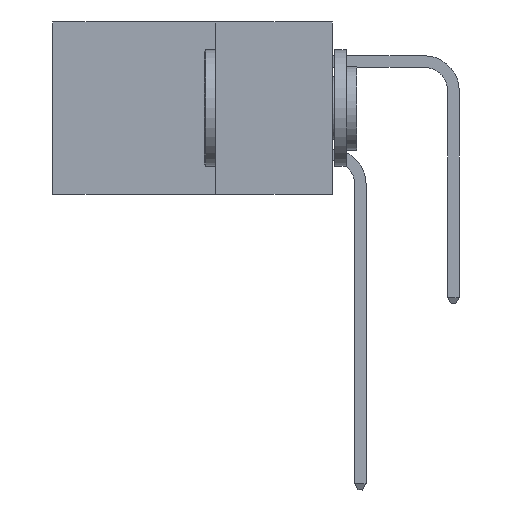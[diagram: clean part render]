
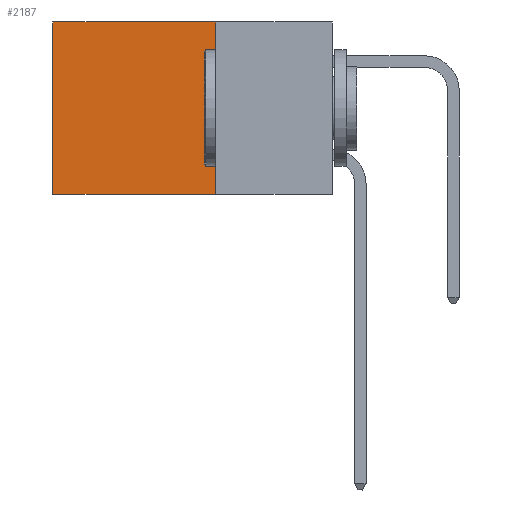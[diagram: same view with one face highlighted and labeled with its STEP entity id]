
A CAD part, left-side view. The second image highlights one B-rep face of the part: STEP entity #2187.
In plain terms, the highlighted planar face has unit normal (-1, 0, 0).
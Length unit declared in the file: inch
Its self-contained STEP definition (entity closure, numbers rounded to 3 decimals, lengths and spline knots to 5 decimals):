
#145 = DIRECTION ( 'NONE',  ( 0., 0., -1. ) ) ;
#839 = VERTEX_POINT ( 'NONE', #13730 ) ;
#934 = EDGE_CURVE ( 'NONE', #3153, #12391, #12369, .T. ) ;
#1310 = CARTESIAN_POINT ( 'NONE',  ( 0.298, 0.6, 0. ) ) ;
#1481 = DIRECTION ( 'NONE',  ( 1., 0., 0. ) ) ;
#1798 = LINE ( 'NONE', #10768, #3981 ) ;
#2094 = EDGE_LOOP ( 'NONE', ( #11423, #9813, #8148, #8895 ) ) ;
#2187 = ADVANCED_FACE ( 'NONE', ( #8051 ), #3829, .F. ) ;
#2209 = DIRECTION ( 'NONE',  ( 0., 1., 0. ) ) ;
#2402 = VECTOR ( 'NONE', #2209, 39.37008 ) ;
#2770 = VECTOR ( 'NONE', #9827, 39.37008 ) ;
#2949 = LINE ( 'NONE', #1310, #2770 ) ;
#3153 = VERTEX_POINT ( 'NONE', #14128 ) ;
#3829 = PLANE ( 'NONE',  #6650 ) ;
#3981 = VECTOR ( 'NONE', #145, 39.37008 ) ;
#4525 = CARTESIAN_POINT ( 'NONE',  ( 0.298, 0.25, -0.37 ) ) ;
#6087 = DIRECTION ( 'NONE',  ( 0., 0., -1. ) ) ;
#6650 = AXIS2_PLACEMENT_3D ( 'NONE', #9384, #1481, #6087 ) ;
#7621 = CARTESIAN_POINT ( 'NONE',  ( 0.298, 0.6, 0. ) ) ;
#8051 = FACE_OUTER_BOUND ( 'NONE', #2094, .T. ) ;
#8148 = ORIENTED_EDGE ( 'NONE', *, *, #14151, .F. ) ;
#8493 = DIRECTION ( 'NONE',  ( 0., 1., 0. ) ) ;
#8543 = CARTESIAN_POINT ( 'NONE',  ( 0.298, 0.25, -0.37 ) ) ;
#8895 = ORIENTED_EDGE ( 'NONE', *, *, #934, .T. ) ;
#9384 = CARTESIAN_POINT ( 'NONE',  ( 0.298, 0.25, 0. ) ) ;
#9813 = ORIENTED_EDGE ( 'NONE', *, *, #10863, .F. ) ;
#9827 = DIRECTION ( 'NONE',  ( 0., 0., -1. ) ) ;
#10152 = EDGE_CURVE ( 'NONE', #12391, #839, #2949, .T. ) ;
#10335 = LINE ( 'NONE', #8543, #13404 ) ;
#10768 = CARTESIAN_POINT ( 'NONE',  ( 0.298, 0.25, 0. ) ) ;
#10863 = EDGE_CURVE ( 'NONE', #12750, #839, #10335, .T. ) ;
#11423 = ORIENTED_EDGE ( 'NONE', *, *, #10152, .T. ) ;
#11540 = CARTESIAN_POINT ( 'NONE',  ( 0.298, 0.25, 0. ) ) ;
#12369 = LINE ( 'NONE', #11540, #2402 ) ;
#12391 = VERTEX_POINT ( 'NONE', #7621 ) ;
#12750 = VERTEX_POINT ( 'NONE', #4525 ) ;
#13404 = VECTOR ( 'NONE', #8493, 39.37008 ) ;
#13730 = CARTESIAN_POINT ( 'NONE',  ( 0.298, 0.6, -0.37 ) ) ;
#14128 = CARTESIAN_POINT ( 'NONE',  ( 0.298, 0.25, 0. ) ) ;
#14151 = EDGE_CURVE ( 'NONE', #3153, #12750, #1798, .T. ) ;
